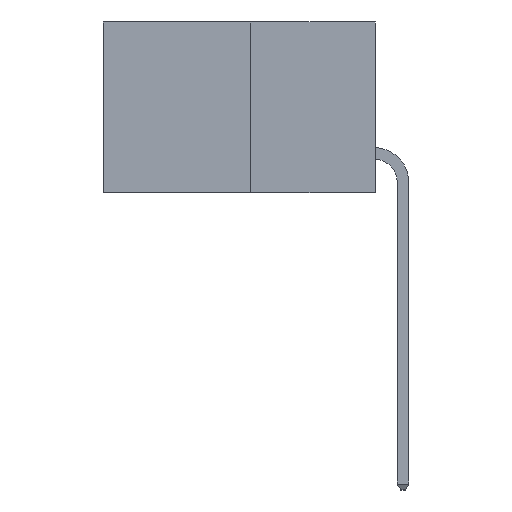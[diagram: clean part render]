
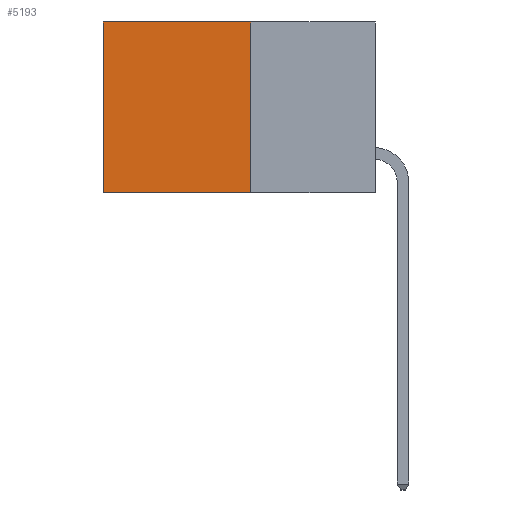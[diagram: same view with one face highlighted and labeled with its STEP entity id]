
A CAD part, left-side view. The second image highlights one B-rep face of the part: STEP entity #5193.
In plain terms, the highlighted planar face has unit normal (-1, 0, 0).
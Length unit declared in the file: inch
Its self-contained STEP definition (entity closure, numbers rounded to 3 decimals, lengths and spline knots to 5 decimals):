
#105 = FACE_OUTER_BOUND ( 'NONE', #1037, .T. ) ;
#399 = EDGE_CURVE ( 'NONE', #7125, #2822, #450, .T. ) ;
#450 = LINE ( 'NONE', #3469, #7669 ) ;
#768 = VECTOR ( 'NONE', #2337, 39.37008 ) ;
#1037 = EDGE_LOOP ( 'NONE', ( #3145, #6406, #7751, #8250 ) ) ;
#1066 = VERTEX_POINT ( 'NONE', #3746 ) ;
#1373 = LINE ( 'NONE', #3081, #8881 ) ;
#2337 = DIRECTION ( 'NONE',  ( 0., 1., 0. ) ) ;
#2427 = VERTEX_POINT ( 'NONE', #8306 ) ;
#2462 = CARTESIAN_POINT ( 'NONE',  ( 0.277, 0.27, 0. ) ) ;
#2652 = DIRECTION ( 'NONE',  ( 0., 1., 0. ) ) ;
#2822 = VERTEX_POINT ( 'NONE', #4959 ) ;
#2863 = CARTESIAN_POINT ( 'NONE',  ( 0.277, 0.27, -0.37 ) ) ;
#3014 = DIRECTION ( 'NONE',  ( 0., 0., -1. ) ) ;
#3081 = CARTESIAN_POINT ( 'NONE',  ( 0.277, 0.27, -0.37 ) ) ;
#3145 = ORIENTED_EDGE ( 'NONE', *, *, #399, .T. ) ;
#3202 = CARTESIAN_POINT ( 'NONE',  ( 0.277, 0.59, 0. ) ) ;
#3214 = EDGE_CURVE ( 'NONE', #2427, #2822, #8369, .T. ) ;
#3469 = CARTESIAN_POINT ( 'NONE',  ( 0.277, 0.59, -0.37 ) ) ;
#3695 = EDGE_CURVE ( 'NONE', #1066, #7125, #8167, .T. ) ;
#3746 = CARTESIAN_POINT ( 'NONE',  ( 0.277, 0.27, 0. ) ) ;
#4104 = DIRECTION ( 'NONE',  ( 0., 0., -1. ) ) ;
#4156 = DIRECTION ( 'NONE',  ( 1., 0., 0. ) ) ;
#4397 = AXIS2_PLACEMENT_3D ( 'NONE', #4453, #4156, #4104 ) ;
#4453 = CARTESIAN_POINT ( 'NONE',  ( 0.277, 0.27, -0.37 ) ) ;
#4480 = PLANE ( 'NONE',  #4397 ) ;
#4631 = VECTOR ( 'NONE', #2652, 39.37008 ) ;
#4897 = DIRECTION ( 'NONE',  ( 0., 0., -1. ) ) ;
#4959 = CARTESIAN_POINT ( 'NONE',  ( 0.277, 0.59, -0.37 ) ) ;
#5193 = ADVANCED_FACE ( 'NONE', ( #105 ), #4480, .F. ) ;
#6406 = ORIENTED_EDGE ( 'NONE', *, *, #3214, .F. ) ;
#7125 = VERTEX_POINT ( 'NONE', #3202 ) ;
#7669 = VECTOR ( 'NONE', #4897, 39.37008 ) ;
#7751 = ORIENTED_EDGE ( 'NONE', *, *, #8215, .F. ) ;
#8167 = LINE ( 'NONE', #2462, #768 ) ;
#8215 = EDGE_CURVE ( 'NONE', #1066, #2427, #1373, .T. ) ;
#8250 = ORIENTED_EDGE ( 'NONE', *, *, #3695, .T. ) ;
#8306 = CARTESIAN_POINT ( 'NONE',  ( 0.277, 0.27, -0.37 ) ) ;
#8369 = LINE ( 'NONE', #2863, #4631 ) ;
#8881 = VECTOR ( 'NONE', #3014, 39.37008 ) ;
